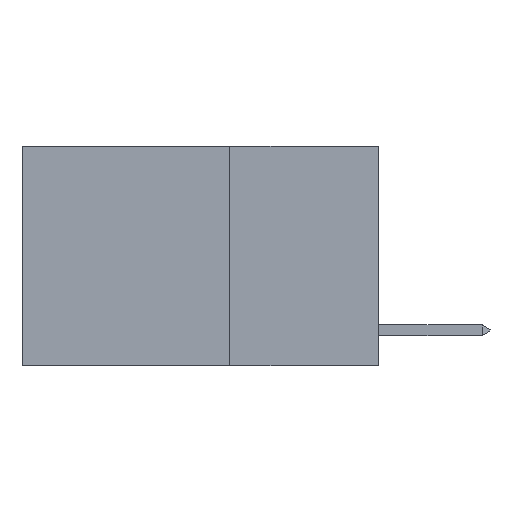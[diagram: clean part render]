
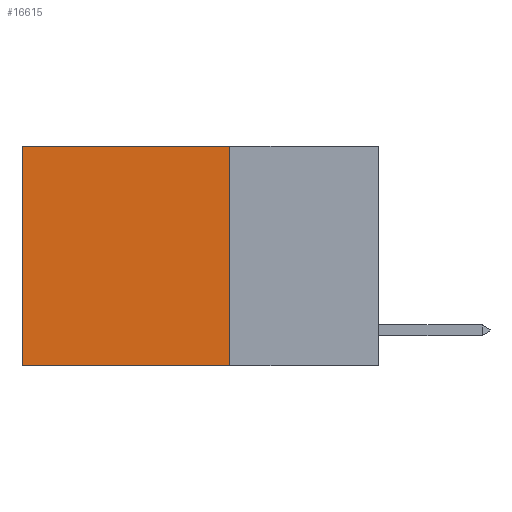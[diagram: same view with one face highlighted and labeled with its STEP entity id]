
A CAD part, left-side view. The second image highlights one B-rep face of the part: STEP entity #16615.
In plain terms, the highlighted planar face has unit normal (-1, 0, 0).
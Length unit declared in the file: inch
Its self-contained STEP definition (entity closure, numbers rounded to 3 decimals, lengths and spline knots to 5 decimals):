
#1248 = DIRECTION ( 'NONE',  ( 0., 0., -1. ) ) ;
#2083 = ORIENTED_EDGE ( 'NONE', *, *, #9597, .F. ) ;
#3446 = VERTEX_POINT ( 'NONE', #17462 ) ;
#4464 = CARTESIAN_POINT ( 'NONE',  ( 0.2625, 0.6, 0. ) ) ;
#4670 = VECTOR ( 'NONE', #21801, 39.37008 ) ;
#4742 = CARTESIAN_POINT ( 'NONE',  ( 0.2625, 0.25, 0. ) ) ;
#6497 = DIRECTION ( 'NONE',  ( 0., 0., -1. ) ) ;
#6596 = VECTOR ( 'NONE', #17104, 39.37008 ) ;
#9597 = EDGE_CURVE ( 'NONE', #15728, #3446, #22861, .T. ) ;
#10119 = EDGE_CURVE ( 'NONE', #24493, #15728, #20310, .T. ) ;
#10327 = VECTOR ( 'NONE', #6497, 39.37008 ) ;
#10787 = DIRECTION ( 'NONE',  ( 0., 1., 0. ) ) ;
#11005 = VECTOR ( 'NONE', #10787, 39.37008 ) ;
#11105 = VERTEX_POINT ( 'NONE', #12572 ) ;
#11480 = PLANE ( 'NONE',  #11940 ) ;
#11940 = AXIS2_PLACEMENT_3D ( 'NONE', #25667, #13507, #1248 ) ;
#12572 = CARTESIAN_POINT ( 'NONE',  ( 0.2625, 0.6, 0. ) ) ;
#12821 = EDGE_LOOP ( 'NONE', ( #17548, #2083, #24968, #20275 ) ) ;
#13507 = DIRECTION ( 'NONE',  ( 1., 0., 0. ) ) ;
#15081 = CARTESIAN_POINT ( 'NONE',  ( 0.2625, 0.25, -0.37 ) ) ;
#15140 = LINE ( 'NONE', #24986, #11005 ) ;
#15719 = LINE ( 'NONE', #4464, #10327 ) ;
#15728 = VERTEX_POINT ( 'NONE', #18703 ) ;
#16615 = ADVANCED_FACE ( 'NONE', ( #24214 ), #11480, .F. ) ;
#17104 = DIRECTION ( 'NONE',  ( 0., 1., 0. ) ) ;
#17462 = CARTESIAN_POINT ( 'NONE',  ( 0.2625, 0.6, -0.37 ) ) ;
#17548 = ORIENTED_EDGE ( 'NONE', *, *, #20870, .T. ) ;
#18703 = CARTESIAN_POINT ( 'NONE',  ( 0.2625, 0.25, -0.37 ) ) ;
#19655 = EDGE_CURVE ( 'NONE', #24493, #11105, #15140, .T. ) ;
#19755 = CARTESIAN_POINT ( 'NONE',  ( 0.2625, 0.25, 0. ) ) ;
#20275 = ORIENTED_EDGE ( 'NONE', *, *, #19655, .T. ) ;
#20310 = LINE ( 'NONE', #19755, #4670 ) ;
#20870 = EDGE_CURVE ( 'NONE', #11105, #3446, #15719, .T. ) ;
#21801 = DIRECTION ( 'NONE',  ( 0., 0., -1. ) ) ;
#22861 = LINE ( 'NONE', #15081, #6596 ) ;
#24214 = FACE_OUTER_BOUND ( 'NONE', #12821, .T. ) ;
#24493 = VERTEX_POINT ( 'NONE', #4742 ) ;
#24968 = ORIENTED_EDGE ( 'NONE', *, *, #10119, .F. ) ;
#24986 = CARTESIAN_POINT ( 'NONE',  ( 0.2625, 0.25, 0. ) ) ;
#25667 = CARTESIAN_POINT ( 'NONE',  ( 0.2625, 0.25, 0. ) ) ;
